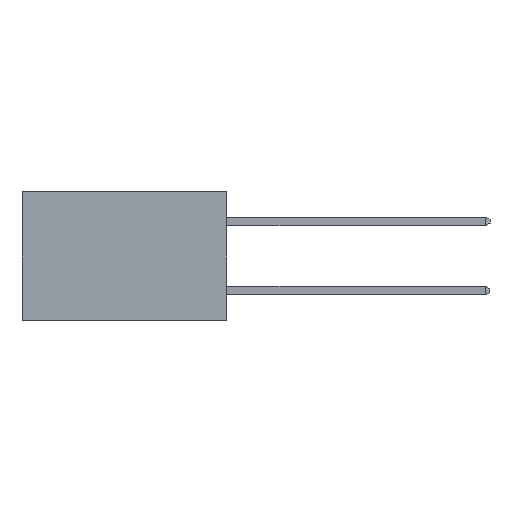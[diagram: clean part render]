
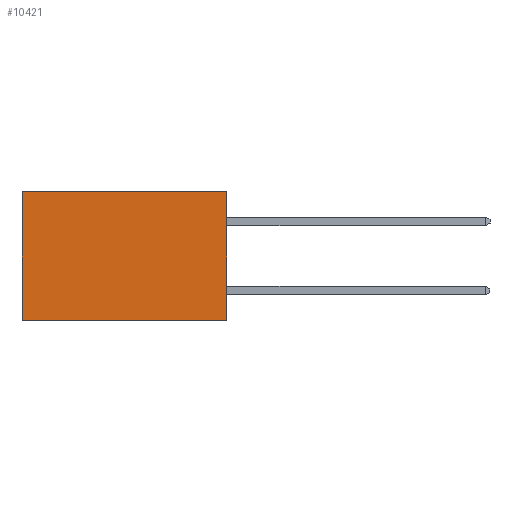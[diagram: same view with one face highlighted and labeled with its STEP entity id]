
A CAD part, left-side view. The second image highlights one B-rep face of the part: STEP entity #10421.
In plain terms, the highlighted planar face has unit normal (-1, 0, 0).
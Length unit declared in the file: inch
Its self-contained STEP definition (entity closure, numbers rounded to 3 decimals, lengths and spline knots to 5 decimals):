
#2187 = VECTOR ( 'NONE', #19958, 39.37008 ) ;
#4073 = ORIENTED_EDGE ( 'NONE', *, *, #27218, .T. ) ;
#5121 = VECTOR ( 'NONE', #18116, 39.37008 ) ;
#6036 = VECTOR ( 'NONE', #29184, 39.37008 ) ;
#6048 = EDGE_CURVE ( 'NONE', #16848, #17819, #24591, .T. ) ;
#9320 = FACE_OUTER_BOUND ( 'NONE', #28418, .T. ) ;
#9579 = CARTESIAN_POINT ( 'NONE',  ( 0.277, 0.59, 0. ) ) ;
#10421 = ADVANCED_FACE ( 'NONE', ( #9320 ), #14544, .F. ) ;
#10598 = LINE ( 'NONE', #25032, #5121 ) ;
#11607 = VECTOR ( 'NONE', #25662, 39.37008 ) ;
#13477 = CARTESIAN_POINT ( 'NONE',  ( 0.277, 0., -0.37 ) ) ;
#13876 = LINE ( 'NONE', #24504, #2187 ) ;
#14161 = EDGE_CURVE ( 'NONE', #16848, #27712, #10598, .T. ) ;
#14275 = DIRECTION ( 'NONE',  ( 0., 0., -1. ) ) ;
#14340 = DIRECTION ( 'NONE',  ( 1., 0., 0. ) ) ;
#14477 = CARTESIAN_POINT ( 'NONE',  ( 0.277, 0., -0.37 ) ) ;
#14544 = PLANE ( 'NONE',  #17977 ) ;
#15785 = ORIENTED_EDGE ( 'NONE', *, *, #26263, .F. ) ;
#16848 = VERTEX_POINT ( 'NONE', #27309 ) ;
#17589 = VERTEX_POINT ( 'NONE', #18197 ) ;
#17819 = VERTEX_POINT ( 'NONE', #9579 ) ;
#17873 = LINE ( 'NONE', #23358, #11607 ) ;
#17977 = AXIS2_PLACEMENT_3D ( 'NONE', #14477, #14340, #14275 ) ;
#18116 = DIRECTION ( 'NONE',  ( 0., 0., -1. ) ) ;
#18197 = CARTESIAN_POINT ( 'NONE',  ( 0.277, 0.59, -0.37 ) ) ;
#19958 = DIRECTION ( 'NONE',  ( 0., 1., 0. ) ) ;
#21703 = ORIENTED_EDGE ( 'NONE', *, *, #6048, .T. ) ;
#23358 = CARTESIAN_POINT ( 'NONE',  ( 0.277, 0.59, -0.37 ) ) ;
#24504 = CARTESIAN_POINT ( 'NONE',  ( 0.277, 0., -0.37 ) ) ;
#24591 = LINE ( 'NONE', #29311, #6036 ) ;
#25032 = CARTESIAN_POINT ( 'NONE',  ( 0.277, 0., -0.37 ) ) ;
#25662 = DIRECTION ( 'NONE',  ( 0., 0., -1. ) ) ;
#26263 = EDGE_CURVE ( 'NONE', #27712, #17589, #13876, .T. ) ;
#27218 = EDGE_CURVE ( 'NONE', #17819, #17589, #17873, .T. ) ;
#27309 = CARTESIAN_POINT ( 'NONE',  ( 0.277, 0., 0. ) ) ;
#27712 = VERTEX_POINT ( 'NONE', #13477 ) ;
#28418 = EDGE_LOOP ( 'NONE', ( #4073, #15785, #28950, #21703 ) ) ;
#28950 = ORIENTED_EDGE ( 'NONE', *, *, #14161, .F. ) ;
#29184 = DIRECTION ( 'NONE',  ( 0., 1., 0. ) ) ;
#29311 = CARTESIAN_POINT ( 'NONE',  ( 0.277, 0., 0. ) ) ;
